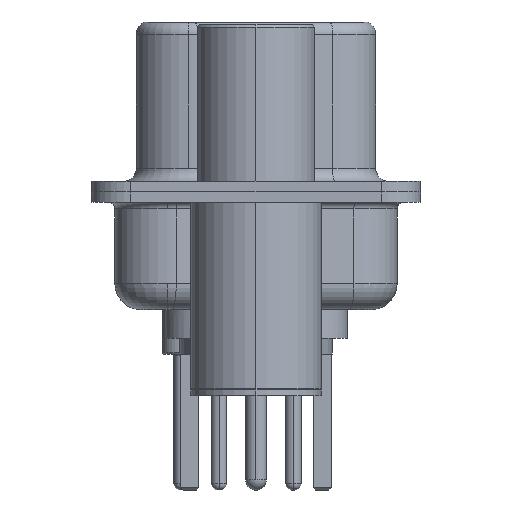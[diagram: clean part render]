
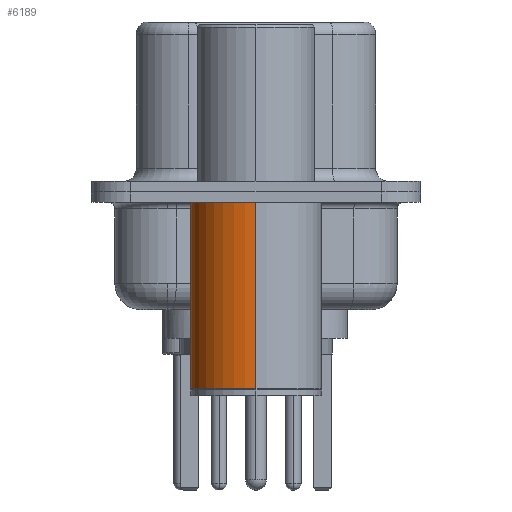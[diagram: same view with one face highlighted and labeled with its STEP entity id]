
A CAD part, left-side view. The second image highlights one B-rep face of the part: STEP entity #6189.
In plain terms, the highlighted cylindrical face has radius 2.5 mm (diameter 5 mm), a partial arc.
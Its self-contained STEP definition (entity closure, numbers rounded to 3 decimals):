
#342 = ORIENTED_EDGE ( 'NONE', *, *, #13029, .T. ) ;
#887 = DIRECTION ( 'NONE',  ( 0., 0., 1. ) ) ;
#890 = CYLINDRICAL_SURFACE ( 'NONE', #4051, 2.5 ) ;
#945 = ORIENTED_EDGE ( 'NONE', *, *, #3204, .F. ) ;
#1631 = CARTESIAN_POINT ( 'NONE',  ( 0., 0., 0.581 ) ) ;
#2176 = EDGE_CURVE ( 'NONE', #18971, #20966, #22315, .T. ) ;
#3204 = EDGE_CURVE ( 'NONE', #25578, #18971, #21220, .T. ) ;
#4051 = AXIS2_PLACEMENT_3D ( 'NONE', #1631, #13488, #23046 ) ;
#5066 = DIRECTION ( 'NONE',  ( 1., 0., 0. ) ) ;
#5419 = AXIS2_PLACEMENT_3D ( 'NONE', #15788, #27956, #16497 ) ;
#6181 = EDGE_LOOP ( 'NONE', ( #21475, #342, #14850, #945 ) ) ;
#6189 = ADVANCED_FACE ( 'NONE', ( #29057 ), #890, .T. ) ;
#7325 = CARTESIAN_POINT ( 'NONE',  ( -2.5, 0., -0.4 ) ) ;
#7465 = VERTEX_POINT ( 'NONE', #22475 ) ;
#13029 = EDGE_CURVE ( 'NONE', #7465, #20966, #18005, .T. ) ;
#13461 = CIRCLE ( 'NONE', #19892, 2.5 ) ;
#13488 = DIRECTION ( 'NONE',  ( 0., 0., 1. ) ) ;
#13920 = CARTESIAN_POINT ( 'NONE',  ( -2.5, 0., 0.581 ) ) ;
#14850 = ORIENTED_EDGE ( 'NONE', *, *, #2176, .F. ) ;
#15788 = CARTESIAN_POINT ( 'NONE',  ( 0., 0., -0.4 ) ) ;
#16497 = DIRECTION ( 'NONE',  ( 1., 0., 0. ) ) ;
#18005 = LINE ( 'NONE', #13920, #24871 ) ;
#18723 = DIRECTION ( 'NONE',  ( 0., 0., 1. ) ) ;
#18971 = VERTEX_POINT ( 'NONE', #28993 ) ;
#19892 = AXIS2_PLACEMENT_3D ( 'NONE', #28340, #887, #5066 ) ;
#20966 = VERTEX_POINT ( 'NONE', #7325 ) ;
#21220 = LINE ( 'NONE', #22173, #28861 ) ;
#21475 = ORIENTED_EDGE ( 'NONE', *, *, #23293, .T. ) ;
#22173 = CARTESIAN_POINT ( 'NONE',  ( 2.5, 0., 0.581 ) ) ;
#22315 = CIRCLE ( 'NONE', #5419, 2.5 ) ;
#22475 = CARTESIAN_POINT ( 'NONE',  ( -2.5, 0., -7.525 ) ) ;
#23046 = DIRECTION ( 'NONE',  ( 1., 0., 0. ) ) ;
#23293 = EDGE_CURVE ( 'NONE', #25578, #7465, #13461, .T. ) ;
#24588 = DIRECTION ( 'NONE',  ( 0., 0., 1. ) ) ;
#24871 = VECTOR ( 'NONE', #18723, 1000. ) ;
#25578 = VERTEX_POINT ( 'NONE', #30130 ) ;
#27956 = DIRECTION ( 'NONE',  ( 0., 0., 1. ) ) ;
#28340 = CARTESIAN_POINT ( 'NONE',  ( 0., 0., -7.525 ) ) ;
#28861 = VECTOR ( 'NONE', #24588, 1000. ) ;
#28993 = CARTESIAN_POINT ( 'NONE',  ( 2.5, 0., -0.4 ) ) ;
#29057 = FACE_OUTER_BOUND ( 'NONE', #6181, .T. ) ;
#30130 = CARTESIAN_POINT ( 'NONE',  ( 2.5, 0., -7.525 ) ) ;
